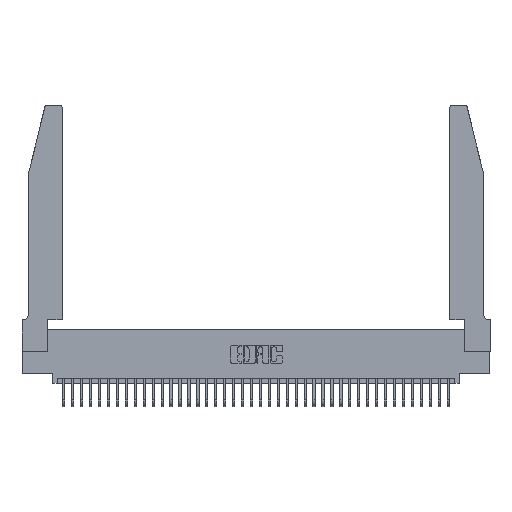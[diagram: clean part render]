
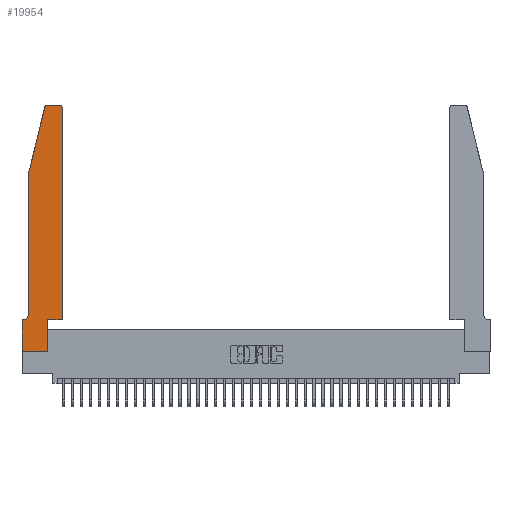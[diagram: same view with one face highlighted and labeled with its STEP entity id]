
A CAD part, top view. The second image highlights one B-rep face of the part: STEP entity #19954.
In plain terms, the highlighted planar face has unit normal (0, 0, 1).
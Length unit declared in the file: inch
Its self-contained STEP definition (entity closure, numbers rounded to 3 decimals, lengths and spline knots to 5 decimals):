
#474 = CARTESIAN_POINT ( 'NONE',  ( 0.4505, 0.35, 0.37 ) ) ;
#1394 = DIRECTION ( 'NONE',  ( 0., -1., 0. ) ) ;
#1686 = ORIENTED_EDGE ( 'NONE', *, *, #32775, .T. ) ;
#2176 = EDGE_CURVE ( 'NONE', #32755, #16999, #29910, .T. ) ;
#2352 = VERTEX_POINT ( 'NONE', #34620 ) ;
#2546 = CARTESIAN_POINT ( 'NONE',  ( 0.284, 2.72, 0.37 ) ) ;
#3692 = DIRECTION ( 'NONE',  ( 1., 0., 0. ) ) ;
#4008 = ORIENTED_EDGE ( 'NONE', *, *, #24662, .T. ) ;
#4069 = VERTEX_POINT ( 'NONE', #30757 ) ;
#4307 = EDGE_LOOP ( 'NONE', ( #4993, #15642, #1686, #26320, #30675, #39546, #28280, #20185, #16085, #7619, #17581, #4008 ) ) ;
#4486 = VERTEX_POINT ( 'NONE', #35906 ) ;
#4566 = CARTESIAN_POINT ( 'NONE',  ( 0.0055, 0.35, 0.37 ) ) ;
#4993 = ORIENTED_EDGE ( 'NONE', *, *, #12013, .T. ) ;
#5042 = VERTEX_POINT ( 'NONE', #4566 ) ;
#5741 = DIRECTION ( 'NONE',  ( 1., 0., 0. ) ) ;
#6006 = PLANE ( 'NONE',  #8410 ) ;
#6679 = VECTOR ( 'NONE', #15002, 39.37008 ) ;
#6895 = EDGE_CURVE ( 'NONE', #2352, #5042, #36493, .T. ) ;
#7295 = CARTESIAN_POINT ( 'NONE',  ( 0.4205, 2.72, 0.37 ) ) ;
#7619 = ORIENTED_EDGE ( 'NONE', *, *, #28185, .T. ) ;
#7796 = LINE ( 'NONE', #18429, #22669 ) ;
#8410 = AXIS2_PLACEMENT_3D ( 'NONE', #25000, #28136, #9243 ) ;
#8746 = CIRCLE ( 'NONE', #34113, 0.03 ) ;
#8771 = VERTEX_POINT ( 'NONE', #12353 ) ;
#9243 = DIRECTION ( 'NONE',  ( 1., 0., 0. ) ) ;
#9842 = DIRECTION ( 'NONE',  ( 0., 0., -1. ) ) ;
#10524 = DIRECTION ( 'NONE',  ( 1., 0., 0. ) ) ;
#11365 = DIRECTION ( 'NONE',  ( -0.239, -0.971, 0. ) ) ;
#11589 = CARTESIAN_POINT ( 'NONE',  ( 0.4505, 0.35, 0.37 ) ) ;
#11860 = LINE ( 'NONE', #39140, #27619 ) ;
#12013 = EDGE_CURVE ( 'NONE', #36808, #4486, #13571, .T. ) ;
#12353 = CARTESIAN_POINT ( 'NONE',  ( 0.4505, 2.72, 0.37 ) ) ;
#13015 = CARTESIAN_POINT ( 'NONE',  ( 0.4205, 2.75, 0.37 ) ) ;
#13413 = AXIS2_PLACEMENT_3D ( 'NONE', #2546, #24728, #5741 ) ;
#13571 = LINE ( 'NONE', #39892, #29318 ) ;
#14687 = EDGE_CURVE ( 'NONE', #5042, #31659, #7796, .T. ) ;
#14856 = VECTOR ( 'NONE', #35636, 39.37008 ) ;
#14883 = CARTESIAN_POINT ( 'NONE',  ( 0., 0.35, 0.37 ) ) ;
#15002 = DIRECTION ( 'NONE',  ( 1., 0., 0. ) ) ;
#15372 = CARTESIAN_POINT ( 'NONE',  ( 0.2865, 0.35, 0.37 ) ) ;
#15642 = ORIENTED_EDGE ( 'NONE', *, *, #28608, .T. ) ;
#15789 = EDGE_CURVE ( 'NONE', #28838, #8771, #18199, .T. ) ;
#16085 = ORIENTED_EDGE ( 'NONE', *, *, #26625, .T. ) ;
#16235 = LINE ( 'NONE', #474, #40214 ) ;
#16387 = CARTESIAN_POINT ( 'NONE',  ( 0.25487, 2.72718, 0.37 ) ) ;
#16657 = VECTOR ( 'NONE', #11365, 39.37008 ) ;
#16909 = AXIS2_PLACEMENT_3D ( 'NONE', #28706, #9842, #31865 ) ;
#16999 = VERTEX_POINT ( 'NONE', #17882 ) ;
#17581 = ORIENTED_EDGE ( 'NONE', *, *, #15789, .T. ) ;
#17636 = LINE ( 'NONE', #17731, #16657 ) ;
#17731 = CARTESIAN_POINT ( 'NONE',  ( 0.0755, 2., 0.37 ) ) ;
#17882 = CARTESIAN_POINT ( 'NONE',  ( 0.2865, 0., 0.37 ) ) ;
#18028 = DIRECTION ( 'NONE',  ( -1., 0., 0. ) ) ;
#18199 = LINE ( 'NONE', #11589, #32901 ) ;
#18429 = CARTESIAN_POINT ( 'NONE',  ( 0.0755, 0.35, 0.37 ) ) ;
#18600 = CARTESIAN_POINT ( 'NONE',  ( 0.0755, 2., 0.37 ) ) ;
#19228 = EDGE_CURVE ( 'NONE', #4069, #2352, #38452, .T. ) ;
#19954 = ADVANCED_FACE ( 'NONE', ( #21961 ), #6006, .T. ) ;
#20185 = ORIENTED_EDGE ( 'NONE', *, *, #2176, .T. ) ;
#21961 = FACE_OUTER_BOUND ( 'NONE', #4307, .T. ) ;
#22669 = VECTOR ( 'NONE', #31033, 39.37008 ) ;
#23071 = CARTESIAN_POINT ( 'NONE',  ( 0.4505, 0.35, 0.37 ) ) ;
#23914 = CARTESIAN_POINT ( 'NONE',  ( 0., 0., 0.37 ) ) ;
#24241 = LINE ( 'NONE', #38769, #14856 ) ;
#24662 = EDGE_CURVE ( 'NONE', #8771, #36808, #8746, .T. ) ;
#24728 = DIRECTION ( 'NONE',  ( 0., 0., 1. ) ) ;
#25000 = CARTESIAN_POINT ( 'NONE',  ( 0., 0.35, 0.37 ) ) ;
#26320 = ORIENTED_EDGE ( 'NONE', *, *, #19228, .T. ) ;
#26625 = EDGE_CURVE ( 'NONE', #16999, #31190, #24241, .T. ) ;
#27155 = EDGE_CURVE ( 'NONE', #31659, #32755, #11860, .T. ) ;
#27619 = VECTOR ( 'NONE', #1394, 39.37008 ) ;
#28136 = DIRECTION ( 'NONE',  ( 0., 0., 1. ) ) ;
#28185 = EDGE_CURVE ( 'NONE', #31190, #28838, #16235, .T. ) ;
#28280 = ORIENTED_EDGE ( 'NONE', *, *, #27155, .T. ) ;
#28608 = EDGE_CURVE ( 'NONE', #4486, #36157, #36778, .T. ) ;
#28706 = CARTESIAN_POINT ( 'NONE',  ( 0.0055, 0.42, 0.37 ) ) ;
#28838 = VERTEX_POINT ( 'NONE', #23071 ) ;
#29318 = VECTOR ( 'NONE', #18028, 39.37008 ) ;
#29385 = DIRECTION ( 'NONE',  ( 0., 0., 1. ) ) ;
#29910 = LINE ( 'NONE', #36926, #6679 ) ;
#30675 = ORIENTED_EDGE ( 'NONE', *, *, #6895, .T. ) ;
#30757 = CARTESIAN_POINT ( 'NONE',  ( 0.0755, 2., 0.37 ) ) ;
#31033 = DIRECTION ( 'NONE',  ( -1., 0., 0. ) ) ;
#31190 = VERTEX_POINT ( 'NONE', #15372 ) ;
#31659 = VERTEX_POINT ( 'NONE', #14883 ) ;
#31865 = DIRECTION ( 'NONE',  ( -1., 0., 0. ) ) ;
#32755 = VERTEX_POINT ( 'NONE', #23914 ) ;
#32775 = EDGE_CURVE ( 'NONE', #36157, #4069, #17636, .T. ) ;
#32901 = VECTOR ( 'NONE', #36567, 39.37008 ) ;
#34113 = AXIS2_PLACEMENT_3D ( 'NONE', #7295, #29385, #10524 ) ;
#34620 = CARTESIAN_POINT ( 'NONE',  ( 0.0755, 0.42, 0.37 ) ) ;
#35636 = DIRECTION ( 'NONE',  ( 0., 1., 0. ) ) ;
#35906 = CARTESIAN_POINT ( 'NONE',  ( 0.284, 2.75, 0.37 ) ) ;
#36157 = VERTEX_POINT ( 'NONE', #16387 ) ;
#36493 = CIRCLE ( 'NONE', #16909, 0.07 ) ;
#36567 = DIRECTION ( 'NONE',  ( 0., 1., 0. ) ) ;
#36778 = CIRCLE ( 'NONE', #13413, 0.03 ) ;
#36808 = VERTEX_POINT ( 'NONE', #13015 ) ;
#36926 = CARTESIAN_POINT ( 'NONE',  ( 0., 0., 0.37 ) ) ;
#38452 = LINE ( 'NONE', #18600, #39430 ) ;
#38769 = CARTESIAN_POINT ( 'NONE',  ( 0.2865, 0.35, 0.37 ) ) ;
#39140 = CARTESIAN_POINT ( 'NONE',  ( 0., 0., 0.37 ) ) ;
#39430 = VECTOR ( 'NONE', #40439, 39.37008 ) ;
#39546 = ORIENTED_EDGE ( 'NONE', *, *, #14687, .T. ) ;
#39892 = CARTESIAN_POINT ( 'NONE',  ( 0.2605, 2.75, 0.37 ) ) ;
#40214 = VECTOR ( 'NONE', #3692, 39.37008 ) ;
#40439 = DIRECTION ( 'NONE',  ( 0., -1., 0. ) ) ;
